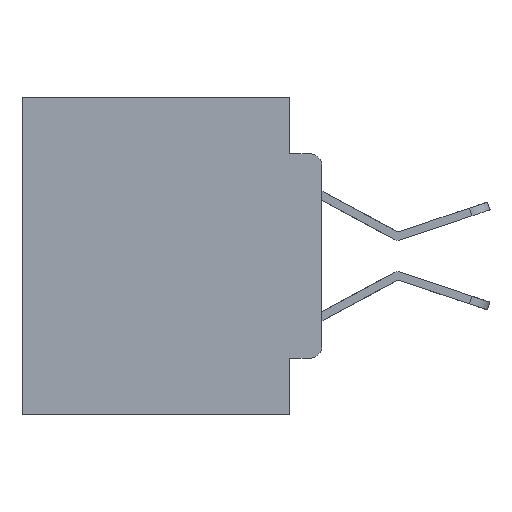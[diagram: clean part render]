
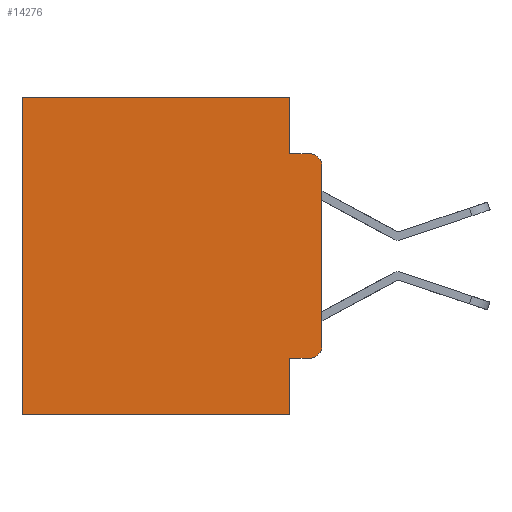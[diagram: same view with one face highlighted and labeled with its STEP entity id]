
A CAD part, left-side view. The second image highlights one B-rep face of the part: STEP entity #14276.
In plain terms, the highlighted planar face has unit normal (-1, 0, 0).
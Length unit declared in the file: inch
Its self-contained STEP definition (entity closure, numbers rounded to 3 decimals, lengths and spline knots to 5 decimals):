
#57 = VERTEX_POINT ( 'NONE', #6537 ) ;
#196 = DIRECTION ( 'NONE',  ( 0., -1., 0. ) ) ;
#420 = CARTESIAN_POINT ( 'NONE',  ( 0.298, 0.473, -0.5 ) ) ;
#516 = EDGE_CURVE ( 'NONE', #10586, #57, #22212, .T. ) ;
#850 = VERTEX_POINT ( 'NONE', #1243 ) ;
#1100 = CARTESIAN_POINT ( 'NONE',  ( 0.298, 0., -0.5 ) ) ;
#1243 = CARTESIAN_POINT ( 'NONE',  ( 0.298, 0., -0.3915 ) ) ;
#2667 = ORIENTED_EDGE ( 'NONE', *, *, #13131, .F. ) ;
#3187 = CARTESIAN_POINT ( 'NONE',  ( 0.298, 0.051, -0.0885 ) ) ;
#4118 = VECTOR ( 'NONE', #20574, 39.37008 ) ;
#4210 = CARTESIAN_POINT ( 'NONE',  ( 0.298, 0., 0. ) ) ;
#4320 = ORIENTED_EDGE ( 'NONE', *, *, #10339, .T. ) ;
#4744 = CARTESIAN_POINT ( 'NONE',  ( 0.298, 0., 0. ) ) ;
#4808 = VERTEX_POINT ( 'NONE', #22108 ) ;
#5256 = VECTOR ( 'NONE', #20264, 39.37008 ) ;
#5622 = DIRECTION ( 'NONE',  ( -1., 0., 0. ) ) ;
#6537 = CARTESIAN_POINT ( 'NONE',  ( 0.298, 0.473, 0. ) ) ;
#6793 = CARTESIAN_POINT ( 'NONE',  ( 0.298, 0.051, -0.0885 ) ) ;
#7169 = CIRCLE ( 'NONE', #14332, 0.02 ) ;
#7439 = ORIENTED_EDGE ( 'NONE', *, *, #8921, .T. ) ;
#7589 = ORIENTED_EDGE ( 'NONE', *, *, #11747, .T. ) ;
#8149 = EDGE_LOOP ( 'NONE', ( #21861, #21268, #17301, #10201, #14046, #7589, #20265, #2667, #4320, #7439 ) ) ;
#8706 = LINE ( 'NONE', #24244, #19162 ) ;
#8921 = EDGE_CURVE ( 'NONE', #4808, #850, #10500, .T. ) ;
#9205 = DIRECTION ( 'NONE',  ( -1., 0., 0. ) ) ;
#9429 = DIRECTION ( 'NONE',  ( 0., 1., 0. ) ) ;
#9901 = CARTESIAN_POINT ( 'NONE',  ( 0.298, 0.051, -0.4115 ) ) ;
#10201 = ORIENTED_EDGE ( 'NONE', *, *, #15921, .F. ) ;
#10316 = CARTESIAN_POINT ( 'NONE',  ( 0.298, 0.051, 0. ) ) ;
#10339 = EDGE_CURVE ( 'NONE', #25470, #4808, #20178, .T. ) ;
#10500 = CIRCLE ( 'NONE', #22179, 0.02 ) ;
#10586 = VERTEX_POINT ( 'NONE', #16910 ) ;
#10785 = VECTOR ( 'NONE', #14560, 39.37008 ) ;
#11258 = PLANE ( 'NONE',  #24489 ) ;
#11438 = CARTESIAN_POINT ( 'NONE',  ( 0.298, 0.051, -0.5 ) ) ;
#11659 = LINE ( 'NONE', #1100, #5256 ) ;
#11747 = EDGE_CURVE ( 'NONE', #57, #12302, #21822, .T. ) ;
#12244 = DIRECTION ( 'NONE',  ( 0., 0., -1. ) ) ;
#12302 = VERTEX_POINT ( 'NONE', #420 ) ;
#12410 = CARTESIAN_POINT ( 'NONE',  ( 0.298, 0.051, -0.4115 ) ) ;
#12465 = CARTESIAN_POINT ( 'NONE',  ( 0.298, 0.473, 0. ) ) ;
#13131 = EDGE_CURVE ( 'NONE', #25470, #25174, #8706, .T. ) ;
#13335 = DIRECTION ( 'NONE',  ( 0., 0., -1. ) ) ;
#13385 = VECTOR ( 'NONE', #196, 39.37008 ) ;
#14046 = ORIENTED_EDGE ( 'NONE', *, *, #516, .T. ) ;
#14051 = LINE ( 'NONE', #6793, #13385 ) ;
#14276 = ADVANCED_FACE ( 'NONE', ( #19144 ), #11258, .F. ) ;
#14332 = AXIS2_PLACEMENT_3D ( 'NONE', #18263, #5622, #20351 ) ;
#14560 = DIRECTION ( 'NONE',  ( 0., 0., -1. ) ) ;
#14656 = VECTOR ( 'NONE', #20353, 39.37008 ) ;
#15921 = EDGE_CURVE ( 'NONE', #10586, #21413, #26970, .T. ) ;
#16910 = CARTESIAN_POINT ( 'NONE',  ( 0.298, 0.051, 0. ) ) ;
#16964 = EDGE_CURVE ( 'NONE', #19360, #17458, #7169, .T. ) ;
#17301 = ORIENTED_EDGE ( 'NONE', *, *, #18707, .F. ) ;
#17379 = VECTOR ( 'NONE', #9429, 39.37008 ) ;
#17458 = VERTEX_POINT ( 'NONE', #17788 ) ;
#17788 = CARTESIAN_POINT ( 'NONE',  ( 0.298, 0.02, -0.0885 ) ) ;
#18263 = CARTESIAN_POINT ( 'NONE',  ( 0.298, 0.02, -0.1085 ) ) ;
#18707 = EDGE_CURVE ( 'NONE', #21413, #17458, #14051, .T. ) ;
#19144 = FACE_OUTER_BOUND ( 'NONE', #8149, .T. ) ;
#19155 = VECTOR ( 'NONE', #12244, 39.37008 ) ;
#19162 = VECTOR ( 'NONE', #26235, 39.37008 ) ;
#19360 = VERTEX_POINT ( 'NONE', #23865 ) ;
#20178 = LINE ( 'NONE', #9901, #14656 ) ;
#20244 = EDGE_CURVE ( 'NONE', #19360, #850, #24608, .T. ) ;
#20264 = DIRECTION ( 'NONE',  ( 0., 1., 0. ) ) ;
#20265 = ORIENTED_EDGE ( 'NONE', *, *, #20804, .F. ) ;
#20351 = DIRECTION ( 'NONE',  ( 0., 0., -1. ) ) ;
#20353 = DIRECTION ( 'NONE',  ( 0., -1., 0. ) ) ;
#20505 = CARTESIAN_POINT ( 'NONE',  ( 0.298, 0., 0. ) ) ;
#20574 = DIRECTION ( 'NONE',  ( 0., 0., -1. ) ) ;
#20804 = EDGE_CURVE ( 'NONE', #25174, #12302, #11659, .T. ) ;
#21268 = ORIENTED_EDGE ( 'NONE', *, *, #16964, .T. ) ;
#21413 = VERTEX_POINT ( 'NONE', #3187 ) ;
#21686 = CARTESIAN_POINT ( 'NONE',  ( 0.298, 0.02, -0.3915 ) ) ;
#21822 = LINE ( 'NONE', #12465, #10785 ) ;
#21861 = ORIENTED_EDGE ( 'NONE', *, *, #20244, .F. ) ;
#22108 = CARTESIAN_POINT ( 'NONE',  ( 0.298, 0.02, -0.4115 ) ) ;
#22179 = AXIS2_PLACEMENT_3D ( 'NONE', #21686, #9205, #23732 ) ;
#22212 = LINE ( 'NONE', #4210, #17379 ) ;
#23732 = DIRECTION ( 'NONE',  ( 0., 0., -1. ) ) ;
#23865 = CARTESIAN_POINT ( 'NONE',  ( 0.298, 0., -0.1085 ) ) ;
#24244 = CARTESIAN_POINT ( 'NONE',  ( 0.298, 0.051, 0. ) ) ;
#24489 = AXIS2_PLACEMENT_3D ( 'NONE', #4744, #25655, #13335 ) ;
#24608 = LINE ( 'NONE', #20505, #19155 ) ;
#25174 = VERTEX_POINT ( 'NONE', #11438 ) ;
#25470 = VERTEX_POINT ( 'NONE', #12410 ) ;
#25655 = DIRECTION ( 'NONE',  ( 1., 0., 0. ) ) ;
#26235 = DIRECTION ( 'NONE',  ( 0., 0., -1. ) ) ;
#26970 = LINE ( 'NONE', #10316, #4118 ) ;
